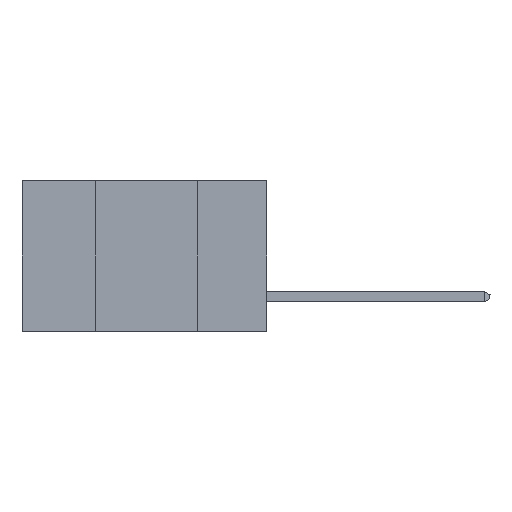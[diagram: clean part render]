
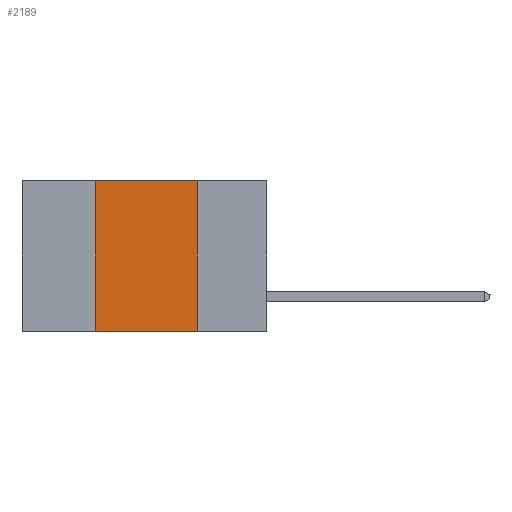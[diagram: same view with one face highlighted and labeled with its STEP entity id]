
A CAD part, left-side view. The second image highlights one B-rep face of the part: STEP entity #2189.
In plain terms, the highlighted planar face has unit normal (-1, 0, 0).
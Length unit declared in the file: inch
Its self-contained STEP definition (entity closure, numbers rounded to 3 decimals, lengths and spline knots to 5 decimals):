
#2189 = ADVANCED_FACE ( 'NONE', ( #10213 ), #5008, .F. ) ;
#2316 = EDGE_CURVE ( 'NONE', #8263, #6688, #16075, .T. ) ;
#3200 = DIRECTION ( 'NONE',  ( 0., 0., -1. ) ) ;
#3591 = CARTESIAN_POINT ( 'NONE',  ( 0., 0.42, -0.37 ) ) ;
#4404 = DIRECTION ( 'NONE',  ( 0., 0., -1. ) ) ;
#4674 = CARTESIAN_POINT ( 'NONE',  ( 0., 0.17, -0.37 ) ) ;
#5008 = PLANE ( 'NONE',  #8877 ) ;
#6111 = CARTESIAN_POINT ( 'NONE',  ( 0., 0.17, 0. ) ) ;
#6337 = VECTOR ( 'NONE', #8951, 39.37008 ) ;
#6688 = VERTEX_POINT ( 'NONE', #4674 ) ;
#7469 = VERTEX_POINT ( 'NONE', #7930 ) ;
#7930 = CARTESIAN_POINT ( 'NONE',  ( 0., 0.42, 0. ) ) ;
#8263 = VERTEX_POINT ( 'NONE', #3591 ) ;
#8877 = AXIS2_PLACEMENT_3D ( 'NONE', #15399, #13708, #3200 ) ;
#8951 = DIRECTION ( 'NONE',  ( 0., -1., 0. ) ) ;
#9164 = EDGE_CURVE ( 'NONE', #13940, #6688, #11186, .T. ) ;
#9231 = VECTOR ( 'NONE', #21873, 39.37008 ) ;
#9838 = CARTESIAN_POINT ( 'NONE',  ( 0., 0.42, 0. ) ) ;
#9995 = EDGE_LOOP ( 'NONE', ( #16847, #14915, #13759, #16444 ) ) ;
#10213 = FACE_OUTER_BOUND ( 'NONE', #9995, .T. ) ;
#11186 = LINE ( 'NONE', #6111, #14197 ) ;
#11307 = DIRECTION ( 'NONE',  ( 0., 0., 1. ) ) ;
#13708 = DIRECTION ( 'NONE',  ( 1., 0., 0. ) ) ;
#13759 = ORIENTED_EDGE ( 'NONE', *, *, #14183, .F. ) ;
#13940 = VERTEX_POINT ( 'NONE', #17619 ) ;
#14183 = EDGE_CURVE ( 'NONE', #8263, #7469, #16610, .T. ) ;
#14197 = VECTOR ( 'NONE', #4404, 39.37008 ) ;
#14915 = ORIENTED_EDGE ( 'NONE', *, *, #15430, .F. ) ;
#15019 = CARTESIAN_POINT ( 'NONE',  ( 0., 0.6, 0. ) ) ;
#15399 = CARTESIAN_POINT ( 'NONE',  ( 0., 0.6, 0. ) ) ;
#15430 = EDGE_CURVE ( 'NONE', #7469, #13940, #18054, .T. ) ;
#16075 = LINE ( 'NONE', #21234, #6337 ) ;
#16444 = ORIENTED_EDGE ( 'NONE', *, *, #2316, .T. ) ;
#16610 = LINE ( 'NONE', #9838, #21043 ) ;
#16847 = ORIENTED_EDGE ( 'NONE', *, *, #9164, .F. ) ;
#17619 = CARTESIAN_POINT ( 'NONE',  ( 0., 0.17, 0. ) ) ;
#18054 = LINE ( 'NONE', #15019, #9231 ) ;
#21043 = VECTOR ( 'NONE', #11307, 39.37008 ) ;
#21234 = CARTESIAN_POINT ( 'NONE',  ( 0., 0.6, -0.37 ) ) ;
#21873 = DIRECTION ( 'NONE',  ( 0., -1., 0. ) ) ;
